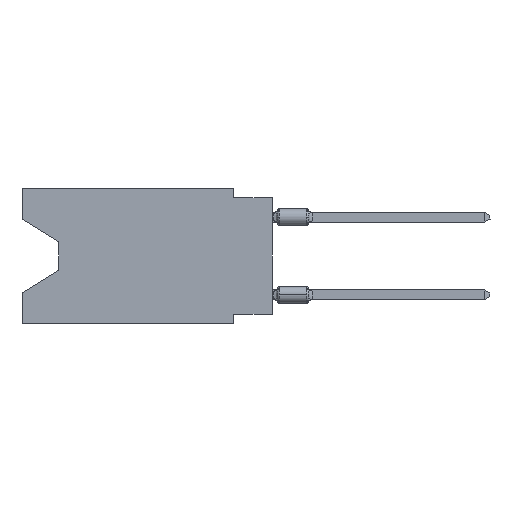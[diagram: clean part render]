
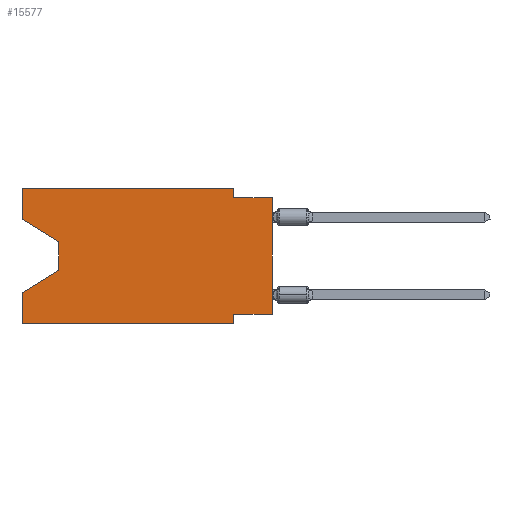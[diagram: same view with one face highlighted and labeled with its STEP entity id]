
A CAD part, left-side view. The second image highlights one B-rep face of the part: STEP entity #15577.
In plain terms, the highlighted planar face has unit normal (-1, 0, 0).
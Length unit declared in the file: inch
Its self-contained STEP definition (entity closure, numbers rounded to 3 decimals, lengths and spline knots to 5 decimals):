
#856 = VERTEX_POINT ( 'NONE', #14205 ) ;
#1490 = LINE ( 'NONE', #55717, #55707 ) ;
#1634 = EDGE_CURVE ( 'NONE', #43450, #42926, #25210, .T. ) ;
#1949 = CARTESIAN_POINT ( 'NONE',  ( 0., 0.55, -0.138 ) ) ;
#1956 = EDGE_CURVE ( 'NONE', #68696, #43450, #44801, .T. ) ;
#2705 = CARTESIAN_POINT ( 'NONE',  ( 0., 0.1, -0.35 ) ) ;
#2953 = DIRECTION ( 'NONE',  ( 0., -1., 0. ) ) ;
#4345 = VECTOR ( 'NONE', #64386, 39.37008 ) ;
#4800 = CARTESIAN_POINT ( 'NONE',  ( 0., 0.645, 0. ) ) ;
#5167 = PLANE ( 'NONE',  #62039 ) ;
#5589 = ORIENTED_EDGE ( 'NONE', *, *, #60446, .F. ) ;
#5736 = CARTESIAN_POINT ( 'NONE',  ( 0., 0.1, 0. ) ) ;
#5882 = DIRECTION ( 'NONE',  ( 1., 0., 0. ) ) ;
#6002 = LINE ( 'NONE', #55234, #44336 ) ;
#6350 = CARTESIAN_POINT ( 'NONE',  ( 0., 0.645, -0.08025 ) ) ;
#6511 = CARTESIAN_POINT ( 'NONE',  ( 0., 0.1, 0. ) ) ;
#8403 = LINE ( 'NONE', #2705, #18923 ) ;
#9004 = CARTESIAN_POINT ( 'NONE',  ( 0., 0., -0.025 ) ) ;
#9078 = VECTOR ( 'NONE', #30062, 39.37008 ) ;
#9508 = ORIENTED_EDGE ( 'NONE', *, *, #13653, .F. ) ;
#10170 = FACE_OUTER_BOUND ( 'NONE', #42814, .T. ) ;
#10568 = EDGE_CURVE ( 'NONE', #66626, #856, #8403, .T. ) ;
#11932 = CARTESIAN_POINT ( 'NONE',  ( 0., 0.55, -0.212 ) ) ;
#12442 = VECTOR ( 'NONE', #36066, 39.37008 ) ;
#12798 = VERTEX_POINT ( 'NONE', #66396 ) ;
#13164 = CARTESIAN_POINT ( 'NONE',  ( 0., 0.645, -0.35 ) ) ;
#13191 = CARTESIAN_POINT ( 'NONE',  ( 0., 0.645, -0.26975 ) ) ;
#13653 = EDGE_CURVE ( 'NONE', #53859, #12798, #51847, .T. ) ;
#13982 = CARTESIAN_POINT ( 'NONE',  ( 0., 0.645, 0. ) ) ;
#14205 = CARTESIAN_POINT ( 'NONE',  ( 0., 0.1, -0.35 ) ) ;
#15176 = CARTESIAN_POINT ( 'NONE',  ( 0., 0.645, 0. ) ) ;
#15320 = ORIENTED_EDGE ( 'NONE', *, *, #37837, .F. ) ;
#15577 = ADVANCED_FACE ( 'NONE', ( #10170 ), #5167, .F. ) ;
#15741 = DIRECTION ( 'NONE',  ( 0., 0., -1. ) ) ;
#16927 = CARTESIAN_POINT ( 'NONE',  ( 0., 0.645, 0. ) ) ;
#17121 = CARTESIAN_POINT ( 'NONE',  ( 0., 0.1, -0.025 ) ) ;
#17281 = LINE ( 'NONE', #50449, #12442 ) ;
#17919 = VERTEX_POINT ( 'NONE', #39019 ) ;
#18266 = DIRECTION ( 'NONE',  ( 0., 0., 1. ) ) ;
#18923 = VECTOR ( 'NONE', #31589, 39.37008 ) ;
#19272 = EDGE_CURVE ( 'NONE', #68341, #42926, #63916, .T. ) ;
#19611 = VERTEX_POINT ( 'NONE', #6511 ) ;
#21495 = VECTOR ( 'NONE', #15741, 39.37008 ) ;
#21573 = LINE ( 'NONE', #16927, #69560 ) ;
#22553 = VERTEX_POINT ( 'NONE', #66863 ) ;
#22838 = ORIENTED_EDGE ( 'NONE', *, *, #1634, .T. ) ;
#24444 = EDGE_CURVE ( 'NONE', #22553, #66626, #17281, .T. ) ;
#25210 = LINE ( 'NONE', #68717, #36462 ) ;
#26960 = DIRECTION ( 'NONE',  ( 0., 0., -1. ) ) ;
#30062 = DIRECTION ( 'NONE',  ( 0., 0., 1. ) ) ;
#31589 = DIRECTION ( 'NONE',  ( 0., 0., -1. ) ) ;
#32296 = LINE ( 'NONE', #4800, #4345 ) ;
#32634 = DIRECTION ( 'NONE',  ( 0., 0., 1. ) ) ;
#32642 = ORIENTED_EDGE ( 'NONE', *, *, #38403, .T. ) ;
#33864 = EDGE_CURVE ( 'NONE', #57246, #68696, #65575, .T. ) ;
#36021 = ORIENTED_EDGE ( 'NONE', *, *, #10568, .F. ) ;
#36066 = DIRECTION ( 'NONE',  ( 0., 1., 0. ) ) ;
#36462 = VECTOR ( 'NONE', #63716, 39.37008 ) ;
#37837 = EDGE_CURVE ( 'NONE', #19611, #53859, #58917, .T. ) ;
#38403 = EDGE_CURVE ( 'NONE', #68341, #856, #6002, .T. ) ;
#39019 = CARTESIAN_POINT ( 'NONE',  ( 0., 0.645, 0. ) ) ;
#40566 = VECTOR ( 'NONE', #66524, 39.37008 ) ;
#42727 = ORIENTED_EDGE ( 'NONE', *, *, #1956, .T. ) ;
#42814 = EDGE_LOOP ( 'NONE', ( #65892, #42727, #22838, #51834, #32642, #36021, #45662, #53244, #9508, #15320, #47074, #5589 ) ) ;
#42926 = VERTEX_POINT ( 'NONE', #13191 ) ;
#42946 = CARTESIAN_POINT ( 'NONE',  ( 0., 0.645, -0.08025 ) ) ;
#43450 = VERTEX_POINT ( 'NONE', #11932 ) ;
#43473 = CARTESIAN_POINT ( 'NONE',  ( 0., 0.55, -0.138 ) ) ;
#44336 = VECTOR ( 'NONE', #60940, 39.37008 ) ;
#44801 = LINE ( 'NONE', #1949, #40566 ) ;
#45662 = ORIENTED_EDGE ( 'NONE', *, *, #24444, .F. ) ;
#47074 = ORIENTED_EDGE ( 'NONE', *, *, #55685, .F. ) ;
#50449 = CARTESIAN_POINT ( 'NONE',  ( 0., 0., -0.325 ) ) ;
#51834 = ORIENTED_EDGE ( 'NONE', *, *, #19272, .F. ) ;
#51847 = LINE ( 'NONE', #9004, #52063 ) ;
#52063 = VECTOR ( 'NONE', #2953, 39.37008 ) ;
#53244 = ORIENTED_EDGE ( 'NONE', *, *, #56164, .T. ) ;
#53859 = VERTEX_POINT ( 'NONE', #17121 ) ;
#53968 = CARTESIAN_POINT ( 'NONE',  ( 0., 0.1, -0.325 ) ) ;
#55234 = CARTESIAN_POINT ( 'NONE',  ( 0., 0.645, -0.35 ) ) ;
#55685 = EDGE_CURVE ( 'NONE', #17919, #19611, #32296, .T. ) ;
#55707 = VECTOR ( 'NONE', #18266, 39.37008 ) ;
#55717 = CARTESIAN_POINT ( 'NONE',  ( 0., 0., 0. ) ) ;
#56164 = EDGE_CURVE ( 'NONE', #22553, #12798, #1490, .T. ) ;
#57246 = VERTEX_POINT ( 'NONE', #42946 ) ;
#58917 = LINE ( 'NONE', #5736, #21495 ) ;
#60446 = EDGE_CURVE ( 'NONE', #57246, #17919, #21573, .T. ) ;
#60940 = DIRECTION ( 'NONE',  ( 0., -1., 0. ) ) ;
#61275 = DIRECTION ( 'NONE',  ( 0., -0.855, -0.519 ) ) ;
#62039 = AXIS2_PLACEMENT_3D ( 'NONE', #15176, #5882, #26960 ) ;
#63716 = DIRECTION ( 'NONE',  ( 0., 0.855, -0.519 ) ) ;
#63916 = LINE ( 'NONE', #13982, #9078 ) ;
#64386 = DIRECTION ( 'NONE',  ( 0., -1., 0. ) ) ;
#65383 = VECTOR ( 'NONE', #61275, 39.37008 ) ;
#65575 = LINE ( 'NONE', #6350, #65383 ) ;
#65892 = ORIENTED_EDGE ( 'NONE', *, *, #33864, .T. ) ;
#66396 = CARTESIAN_POINT ( 'NONE',  ( 0., 0., -0.025 ) ) ;
#66524 = DIRECTION ( 'NONE',  ( 0., 0., -1. ) ) ;
#66626 = VERTEX_POINT ( 'NONE', #53968 ) ;
#66863 = CARTESIAN_POINT ( 'NONE',  ( 0., 0., -0.325 ) ) ;
#68341 = VERTEX_POINT ( 'NONE', #13164 ) ;
#68696 = VERTEX_POINT ( 'NONE', #43473 ) ;
#68717 = CARTESIAN_POINT ( 'NONE',  ( 0., 0.55, -0.212 ) ) ;
#69560 = VECTOR ( 'NONE', #32634, 39.37008 ) ;
